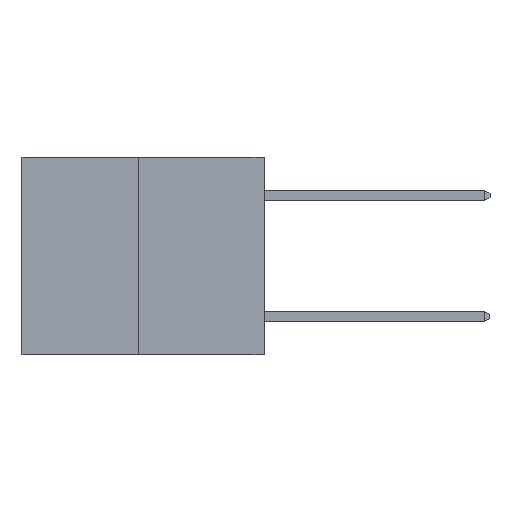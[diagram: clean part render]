
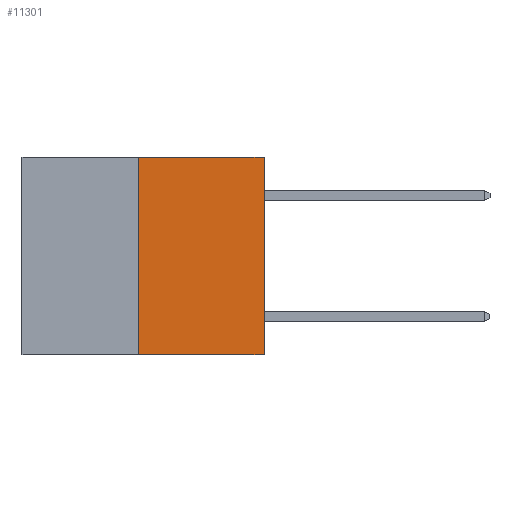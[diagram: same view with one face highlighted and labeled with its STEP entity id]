
A CAD part, left-side view. The second image highlights one B-rep face of the part: STEP entity #11301.
In plain terms, the highlighted planar face has unit normal (-1, 0, 0).
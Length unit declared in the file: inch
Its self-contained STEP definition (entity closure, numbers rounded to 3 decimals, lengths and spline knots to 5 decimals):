
#208 = PLANE ( 'NONE',  #1747 ) ;
#212 = EDGE_LOOP ( 'NONE', ( #15276, #4895, #8334, #5686 ) ) ;
#245 = EDGE_CURVE ( 'NONE', #8185, #1875, #12390, .T. ) ;
#761 = LINE ( 'NONE', #12549, #7850 ) ;
#1548 = DIRECTION ( 'NONE',  ( 0., 0., -1. ) ) ;
#1747 = AXIS2_PLACEMENT_3D ( 'NONE', #7485, #8793, #1548 ) ;
#1875 = VERTEX_POINT ( 'NONE', #4514 ) ;
#2231 = CARTESIAN_POINT ( 'NONE',  ( 0., 0.312, -0.49 ) ) ;
#2444 = VECTOR ( 'NONE', #4109, 39.37008 ) ;
#3028 = EDGE_CURVE ( 'NONE', #11698, #13039, #761, .T. ) ;
#3203 = LINE ( 'NONE', #8023, #2444 ) ;
#3516 = CARTESIAN_POINT ( 'NONE',  ( 0., 0.312, -0.49 ) ) ;
#3661 = DIRECTION ( 'NONE',  ( 0., 0., 1. ) ) ;
#4109 = DIRECTION ( 'NONE',  ( 0., -1., 0. ) ) ;
#4514 = CARTESIAN_POINT ( 'NONE',  ( 0., 0.312, 0. ) ) ;
#4895 = ORIENTED_EDGE ( 'NONE', *, *, #5707, .T. ) ;
#4993 = DIRECTION ( 'NONE',  ( 0., -1., 0. ) ) ;
#5686 = ORIENTED_EDGE ( 'NONE', *, *, #8770, .F. ) ;
#5707 = EDGE_CURVE ( 'NONE', #8185, #11698, #3203, .T. ) ;
#5995 = LINE ( 'NONE', #9899, #14284 ) ;
#7485 = CARTESIAN_POINT ( 'NONE',  ( 0., 0.6, 0. ) ) ;
#7850 = VECTOR ( 'NONE', #13812, 39.37008 ) ;
#8023 = CARTESIAN_POINT ( 'NONE',  ( 0., 0.6, -0.49 ) ) ;
#8185 = VERTEX_POINT ( 'NONE', #3516 ) ;
#8334 = ORIENTED_EDGE ( 'NONE', *, *, #3028, .T. ) ;
#8770 = EDGE_CURVE ( 'NONE', #1875, #13039, #5995, .T. ) ;
#8793 = DIRECTION ( 'NONE',  ( 1., 0., 0. ) ) ;
#9414 = CARTESIAN_POINT ( 'NONE',  ( 0., 0., 0. ) ) ;
#9899 = CARTESIAN_POINT ( 'NONE',  ( 0., 0.6, 0. ) ) ;
#11301 = ADVANCED_FACE ( 'NONE', ( #14506 ), #208, .F. ) ;
#11698 = VERTEX_POINT ( 'NONE', #12676 ) ;
#12390 = LINE ( 'NONE', #2231, #13926 ) ;
#12549 = CARTESIAN_POINT ( 'NONE',  ( 0., 0., 0. ) ) ;
#12676 = CARTESIAN_POINT ( 'NONE',  ( 0., 0., -0.49 ) ) ;
#13039 = VERTEX_POINT ( 'NONE', #9414 ) ;
#13812 = DIRECTION ( 'NONE',  ( 0., 0., 1. ) ) ;
#13926 = VECTOR ( 'NONE', #3661, 39.37008 ) ;
#14284 = VECTOR ( 'NONE', #4993, 39.37008 ) ;
#14506 = FACE_OUTER_BOUND ( 'NONE', #212, .T. ) ;
#15276 = ORIENTED_EDGE ( 'NONE', *, *, #245, .F. ) ;
